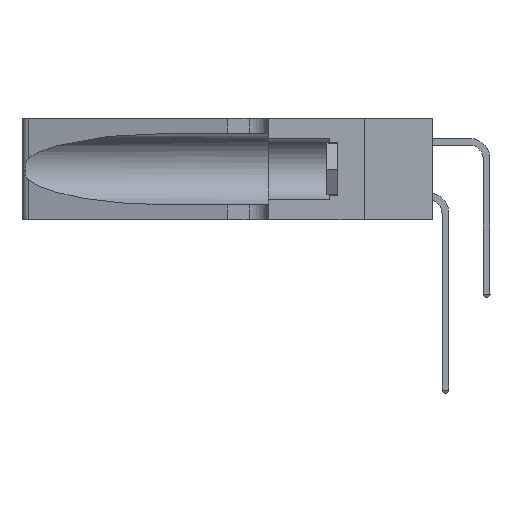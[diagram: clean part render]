
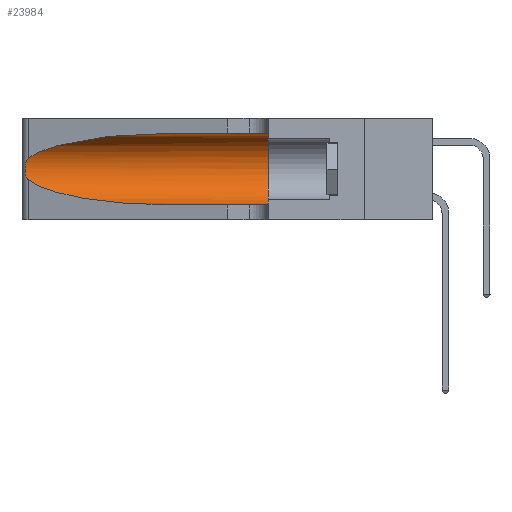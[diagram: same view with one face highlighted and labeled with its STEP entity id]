
A CAD part, left-side view. The second image highlights one B-rep face of the part: STEP entity #23984.
In plain terms, the highlighted cylindrical face has radius 3.308 mm (diameter 6.617 mm), a partial arc.
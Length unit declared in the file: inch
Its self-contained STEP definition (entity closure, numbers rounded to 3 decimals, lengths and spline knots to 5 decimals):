
#2116 =( BOUNDED_CURVE ( )  B_SPLINE_CURVE ( 3, ( #8225, #25734, #31498, #14131 ),
 .UNSPECIFIED., .F., .F. ) 
 B_SPLINE_CURVE_WITH_KNOTS ( ( 4, 4 ),
 ( 3.44316, 4.71239 ),
 .UNSPECIFIED. ) 
 CURVE ( )  GEOMETRIC_REPRESENTATION_ITEM ( )  RATIONAL_B_SPLINE_CURVE ( ( 1., 0.87, 0.87, 1. ) ) 
 REPRESENTATION_ITEM ( '' )  );
#2238 = CARTESIAN_POINT ( 'NONE',  ( 0.26017, 1.23833, 0.17102 ) ) ;
#3019 = EDGE_LOOP ( 'NONE', ( #8415, #5734, #11115, #3238, #14803, #23160 ) ) ;
#3238 = ORIENTED_EDGE ( 'NONE', *, *, #21475, .T. ) ;
#3498 = CARTESIAN_POINT ( 'NONE',  ( 0.1305, 1.61858, 0.05475 ) ) ;
#4816 = VERTEX_POINT ( 'NONE', #8769 ) ;
#5014 = EDGE_CURVE ( 'NONE', #28584, #33488, #11941, .T. ) ;
#5290 = CARTESIAN_POINT ( 'NONE',  ( 0.25789, 1.23486, 0.15765 ) ) ;
#5512 = EDGE_CURVE ( 'NONE', #4816, #12647, #31955, .T. ) ;
#5734 = ORIENTED_EDGE ( 'NONE', *, *, #25544, .T. ) ;
#6132 = VERTEX_POINT ( 'NONE', #11525 ) ;
#6511 = DIRECTION ( 'NONE',  ( 0., -1., 0. ) ) ;
#8225 = CARTESIAN_POINT ( 'NONE',  ( 0.25487, 1.22718, 0.14631 ) ) ;
#8299 = CARTESIAN_POINT ( 'NONE',  ( 0.25555, 1.22993, 0.14849 ) ) ;
#8415 = ORIENTED_EDGE ( 'NONE', *, *, #5014, .T. ) ;
#8557 = CARTESIAN_POINT ( 'NONE',  ( 0.1305, 1.61858, 0.185 ) ) ;
#8769 = CARTESIAN_POINT ( 'NONE',  ( 0.1305, 0.35, 0.31525 ) ) ;
#9152 = DIRECTION ( 'NONE',  ( 0., -1., 0. ) ) ;
#9739 = AXIS2_PLACEMENT_3D ( 'NONE', #8557, #34780, #28955 ) ;
#11115 = ORIENTED_EDGE ( 'NONE', *, *, #16781, .T. ) ;
#11525 = CARTESIAN_POINT ( 'NONE',  ( 0.1305, 0.72297, 0.05475 ) ) ;
#11580 = CYLINDRICAL_SURFACE ( 'NONE', #9739, 0.13025 ) ;
#11941 =( BOUNDED_CURVE ( )  B_SPLINE_CURVE ( 3, ( #32928, #27141, #12504, #15580 ),
 .UNSPECIFIED., .F., .F. ) 
 B_SPLINE_CURVE_WITH_KNOTS ( ( 4, 4 ),
 ( 1.5708, 2.84003 ),
 .UNSPECIFIED. ) 
 CURVE ( )  GEOMETRIC_REPRESENTATION_ITEM ( )  RATIONAL_B_SPLINE_CURVE ( ( 1., 0.87, 0.87, 1. ) ) 
 REPRESENTATION_ITEM ( '' )  );
#12504 = CARTESIAN_POINT ( 'NONE',  ( 0.2373, 1.15595, 0.28018 ) ) ;
#12647 = VERTEX_POINT ( 'NONE', #31342 ) ;
#12652 = CARTESIAN_POINT ( 'NONE',  ( 0.1305, 0.72297, 0.31525 ) ) ;
#13961 = CARTESIAN_POINT ( 'NONE',  ( 0.25555, 1.22994, 0.2215 ) ) ;
#14081 = CARTESIAN_POINT ( 'NONE',  ( 0.25787, 1.23484, 0.2124 ) ) ;
#14131 = CARTESIAN_POINT ( 'NONE',  ( 0.1305, 0.72297, 0.05475 ) ) ;
#14803 = ORIENTED_EDGE ( 'NONE', *, *, #5512, .F. ) ;
#15580 = CARTESIAN_POINT ( 'NONE',  ( 0.25487, 1.22718, 0.22369 ) ) ;
#16781 = EDGE_CURVE ( 'NONE', #27810, #6132, #2116, .T. ) ;
#16982 = CARTESIAN_POINT ( 'NONE',  ( 0.26018, 1.23835, 0.19895 ) ) ;
#17230 = VECTOR ( 'NONE', #9152, 39.37008 ) ;
#17783 = CARTESIAN_POINT ( 'NONE',  ( 0.1305, 0.35, 0.185 ) ) ;
#18149 = LINE ( 'NONE', #23704, #17230 ) ;
#18845 = LINE ( 'NONE', #3498, #33361 ) ;
#19806 = CARTESIAN_POINT ( 'NONE',  ( 0.25487, 1.22718, 0.22369 ) ) ;
#19921 = CARTESIAN_POINT ( 'NONE',  ( 0.26075, 1.23896, 0.178 ) ) ;
#20710 = DIRECTION ( 'NONE',  ( 0., 0., 1. ) ) ;
#21475 = EDGE_CURVE ( 'NONE', #6132, #12647, #18845, .T. ) ;
#21784 = DIRECTION ( 'NONE',  ( 0., 1., 0. ) ) ;
#22849 = CARTESIAN_POINT ( 'NONE',  ( 0.25856, 1.23593, 0.16098 ) ) ;
#23160 = ORIENTED_EDGE ( 'NONE', *, *, #37118, .F. ) ;
#23704 = CARTESIAN_POINT ( 'NONE',  ( 0.1305, 1.61858, 0.31525 ) ) ;
#23984 = ADVANCED_FACE ( 'NONE', ( #31372 ), #11580, .F. ) ;
#25544 = EDGE_CURVE ( 'NONE', #33488, #27810, #30595, .T. ) ;
#25734 = CARTESIAN_POINT ( 'NONE',  ( 0.2373, 1.15595, 0.08982 ) ) ;
#25805 = CARTESIAN_POINT ( 'NONE',  ( 0.25639, 1.23186, 0.15144 ) ) ;
#27141 = CARTESIAN_POINT ( 'NONE',  ( 0.18966, 0.96281, 0.31525 ) ) ;
#27810 = VERTEX_POINT ( 'NONE', #35673 ) ;
#28584 = VERTEX_POINT ( 'NONE', #12652 ) ;
#28711 = CARTESIAN_POINT ( 'NONE',  ( 0.25487, 1.22718, 0.14631 ) ) ;
#28955 = DIRECTION ( 'NONE',  ( 0., 0., -1. ) ) ;
#30595 = B_SPLINE_CURVE_WITH_KNOTS ( 'NONE', 3,
 ( #19806, #13961, #31450, #14081, #34398, #16982, #37347, #19921, #2238, #22849, #5290, #25805, #8299, #28711 ),
 .UNSPECIFIED., .F., .F.,
 ( 4, 2, 2, 2, 2, 2, 4 ),
 ( 0., 0.00027, 0.00053, 0.00107, 0.0016, 0.00187, 0.00214 ),
 .UNSPECIFIED. ) ;
#31342 = CARTESIAN_POINT ( 'NONE',  ( 0.1305, 0.35, 0.05475 ) ) ;
#31372 = FACE_OUTER_BOUND ( 'NONE', #3019, .T. ) ;
#31450 = CARTESIAN_POINT ( 'NONE',  ( 0.25639, 1.23184, 0.21858 ) ) ;
#31498 = CARTESIAN_POINT ( 'NONE',  ( 0.18966, 0.96281, 0.05475 ) ) ;
#31955 = CIRCLE ( 'NONE', #34363, 0.13025 ) ;
#32928 = CARTESIAN_POINT ( 'NONE',  ( 0.1305, 0.72297, 0.31525 ) ) ;
#33361 = VECTOR ( 'NONE', #6511, 39.37008 ) ;
#33488 = VERTEX_POINT ( 'NONE', #35927 ) ;
#34363 = AXIS2_PLACEMENT_3D ( 'NONE', #17783, #21784, #20710 ) ;
#34398 = CARTESIAN_POINT ( 'NONE',  ( 0.25854, 1.2359, 0.20912 ) ) ;
#34780 = DIRECTION ( 'NONE',  ( 0., -1., 0. ) ) ;
#35673 = CARTESIAN_POINT ( 'NONE',  ( 0.25487, 1.22718, 0.14631 ) ) ;
#35927 = CARTESIAN_POINT ( 'NONE',  ( 0.25487, 1.22718, 0.22369 ) ) ;
#37118 = EDGE_CURVE ( 'NONE', #28584, #4816, #18149, .T. ) ;
#37347 = CARTESIAN_POINT ( 'NONE',  ( 0.26075, 1.23896, 0.19203 ) ) ;
